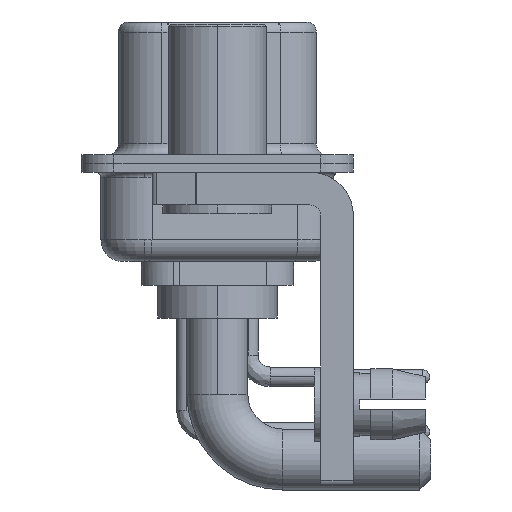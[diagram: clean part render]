
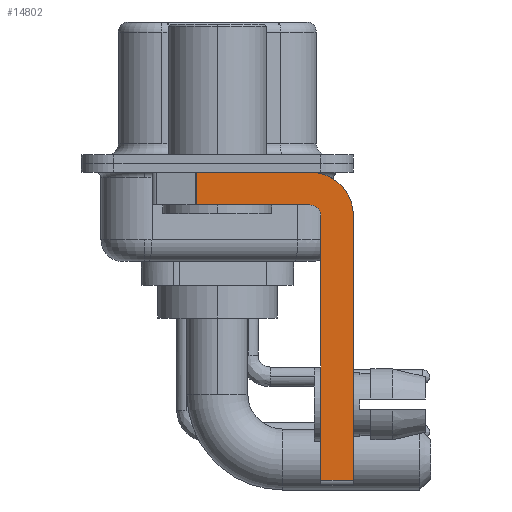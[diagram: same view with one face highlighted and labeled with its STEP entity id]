
A CAD part, left-side view. The second image highlights one B-rep face of the part: STEP entity #14802.
In plain terms, the highlighted planar face has unit normal (-1, 0, 0).
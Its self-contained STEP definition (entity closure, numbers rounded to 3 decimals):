
#809 = PLANE ( 'NONE',  #14163 ) ;
#994 = CARTESIAN_POINT ( 'NONE',  ( -2.9, -4.25, -2.4 ) ) ;
#1351 = VERTEX_POINT ( 'NONE', #6403 ) ;
#1423 = EDGE_CURVE ( 'NONE', #13322, #24882, #3034, .T. ) ;
#2129 = LINE ( 'NONE', #17936, #17365 ) ;
#3034 = LINE ( 'NONE', #7549, #24539 ) ;
#3329 = VERTEX_POINT ( 'NONE', #27609 ) ;
#4168 = ORIENTED_EDGE ( 'NONE', *, *, #6305, .F. ) ;
#4204 = DIRECTION ( 'NONE',  ( 0., -1., 0. ) ) ;
#4806 = DIRECTION ( 'NONE',  ( 0., 1., 0. ) ) ;
#4938 = ORIENTED_EDGE ( 'NONE', *, *, #8455, .F. ) ;
#5086 = VERTEX_POINT ( 'NONE', #24851 ) ;
#5333 = CARTESIAN_POINT ( 'NONE',  ( -2.9, -4.25, -1.9 ) ) ;
#5581 = EDGE_CURVE ( 'NONE', #6816, #21976, #5973, .T. ) ;
#5947 = CIRCLE ( 'NONE', #9646, 0.5 ) ;
#5973 = LINE ( 'NONE', #7852, #6265 ) ;
#6265 = VECTOR ( 'NONE', #14208, 1000. ) ;
#6305 = EDGE_CURVE ( 'NONE', #19522, #1351, #26590, .T. ) ;
#6377 = DIRECTION ( 'NONE',  ( 0., 0., -1. ) ) ;
#6403 = CARTESIAN_POINT ( 'NONE',  ( -2.9, -4.75, -2.4 ) ) ;
#6518 = ORIENTED_EDGE ( 'NONE', *, *, #28457, .F. ) ;
#6816 = VERTEX_POINT ( 'NONE', #25924 ) ;
#7056 = LINE ( 'NONE', #26428, #19886 ) ;
#7405 = ORIENTED_EDGE ( 'NONE', *, *, #19857, .F. ) ;
#7549 = CARTESIAN_POINT ( 'NONE',  ( -2.9, -4.25, -1.9 ) ) ;
#7647 = DIRECTION ( 'NONE',  ( 1., 0., 0. ) ) ;
#7852 = CARTESIAN_POINT ( 'NONE',  ( -2.9, -6.25, -2.4 ) ) ;
#8455 = EDGE_CURVE ( 'NONE', #1351, #13322, #5947, .T. ) ;
#9646 = AXIS2_PLACEMENT_3D ( 'NONE', #21351, #21488, #28124 ) ;
#10576 = ORIENTED_EDGE ( 'NONE', *, *, #5581, .F. ) ;
#11166 = CARTESIAN_POINT ( 'NONE',  ( -2.9, 3., -0.4 ) ) ;
#11851 = FACE_OUTER_BOUND ( 'NONE', #11866, .T. ) ;
#11866 = EDGE_LOOP ( 'NONE', ( #6518, #24130, #20297, #4938, #4168, #27707, #10576, #7405 ) ) ;
#12023 = CARTESIAN_POINT ( 'NONE',  ( -2.9, -4.75, -14.55 ) ) ;
#12084 = DIRECTION ( 'NONE',  ( 0., 0., 1. ) ) ;
#13322 = VERTEX_POINT ( 'NONE', #5333 ) ;
#13328 = LINE ( 'NONE', #11166, #19428 ) ;
#14163 = AXIS2_PLACEMENT_3D ( 'NONE', #27316, #7647, #26135 ) ;
#14208 = DIRECTION ( 'NONE',  ( 0., 0., -1. ) ) ;
#14630 = EDGE_CURVE ( 'NONE', #3329, #24882, #2129, .T. ) ;
#14802 = ADVANCED_FACE ( 'NONE', ( #11851 ), #809, .F. ) ;
#16808 = CARTESIAN_POINT ( 'NONE',  ( -2.9, 0.978, -1.9 ) ) ;
#16970 = VECTOR ( 'NONE', #12084, 1000. ) ;
#17365 = VECTOR ( 'NONE', #24156, 1000. ) ;
#17464 = DIRECTION ( 'NONE',  ( 0., -1., 0. ) ) ;
#17936 = CARTESIAN_POINT ( 'NONE',  ( -2.9, 0.978, -1.9 ) ) ;
#18093 = CARTESIAN_POINT ( 'NONE',  ( -2.9, -6.25, -14.55 ) ) ;
#18972 = CIRCLE ( 'NONE', #22181, 2. ) ;
#19428 = VECTOR ( 'NONE', #4204, 1000. ) ;
#19522 = VERTEX_POINT ( 'NONE', #12023 ) ;
#19857 = EDGE_CURVE ( 'NONE', #5086, #6816, #18972, .T. ) ;
#19886 = VECTOR ( 'NONE', #17464, 1000. ) ;
#20297 = ORIENTED_EDGE ( 'NONE', *, *, #1423, .F. ) ;
#20594 = EDGE_CURVE ( 'NONE', #19522, #21976, #7056, .T. ) ;
#21351 = CARTESIAN_POINT ( 'NONE',  ( -2.9, -4.25, -2.4 ) ) ;
#21488 = DIRECTION ( 'NONE',  ( -1., 0., 0. ) ) ;
#21976 = VERTEX_POINT ( 'NONE', #18093 ) ;
#22181 = AXIS2_PLACEMENT_3D ( 'NONE', #994, #28062, #6377 ) ;
#22268 = CARTESIAN_POINT ( 'NONE',  ( -2.9, -4.75, -14.8 ) ) ;
#24130 = ORIENTED_EDGE ( 'NONE', *, *, #14630, .T. ) ;
#24156 = DIRECTION ( 'NONE',  ( 0., 0., -1. ) ) ;
#24539 = VECTOR ( 'NONE', #4806, 1000. ) ;
#24851 = CARTESIAN_POINT ( 'NONE',  ( -2.9, -4.25, -0.4 ) ) ;
#24882 = VERTEX_POINT ( 'NONE', #16808 ) ;
#25924 = CARTESIAN_POINT ( 'NONE',  ( -2.9, -6.25, -2.4 ) ) ;
#26135 = DIRECTION ( 'NONE',  ( 0., 0., -1. ) ) ;
#26428 = CARTESIAN_POINT ( 'NONE',  ( -2.9, -4.25, -14.55 ) ) ;
#26590 = LINE ( 'NONE', #22268, #16970 ) ;
#27316 = CARTESIAN_POINT ( 'NONE',  ( -2.9, -4.25, -2.4 ) ) ;
#27609 = CARTESIAN_POINT ( 'NONE',  ( -2.9, 0.978, -0.4 ) ) ;
#27707 = ORIENTED_EDGE ( 'NONE', *, *, #20594, .T. ) ;
#28062 = DIRECTION ( 'NONE',  ( 1., 0., 0. ) ) ;
#28124 = DIRECTION ( 'NONE',  ( 0., 0., 1. ) ) ;
#28457 = EDGE_CURVE ( 'NONE', #3329, #5086, #13328, .T. ) ;
